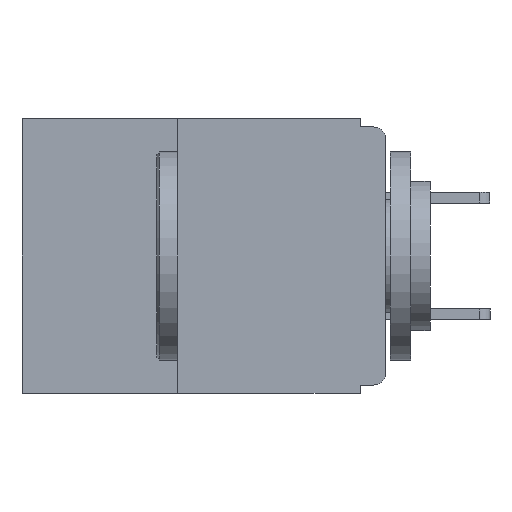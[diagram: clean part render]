
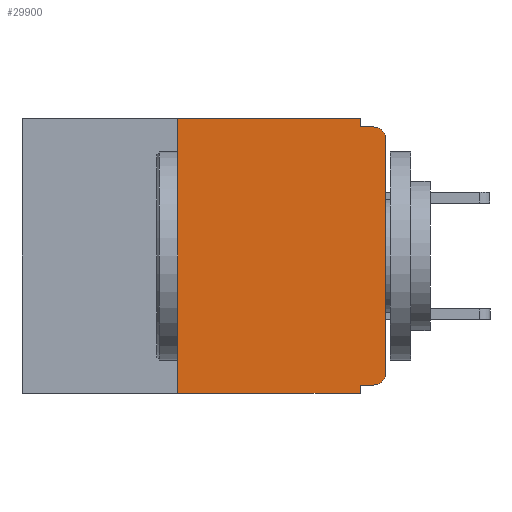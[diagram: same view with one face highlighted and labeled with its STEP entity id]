
A CAD part, left-side view. The second image highlights one B-rep face of the part: STEP entity #29900.
In plain terms, the highlighted planar face has unit normal (-1, 0, 0).
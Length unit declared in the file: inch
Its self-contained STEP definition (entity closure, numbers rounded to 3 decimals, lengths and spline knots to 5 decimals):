
#8 = CARTESIAN_POINT ( 'NONE',  ( 0., 0.031, -0.01 ) ) ;
#133 = CARTESIAN_POINT ( 'NONE',  ( 0., 0.031, 0. ) ) ;
#353 = CARTESIAN_POINT ( 'NONE',  ( 0., 0.437, 0. ) ) ;
#1776 = LINE ( 'NONE', #27268, #23215 ) ;
#1921 = EDGE_CURVE ( 'NONE', #31003, #8344, #16823, .T. ) ;
#2212 = LINE ( 'NONE', #31842, #16308 ) ;
#3171 = AXIS2_PLACEMENT_3D ( 'NONE', #21907, #5169, #24621 ) ;
#3263 = DIRECTION ( 'NONE',  ( 0., -1., 0. ) ) ;
#4074 = VERTEX_POINT ( 'NONE', #21590 ) ;
#4586 = CARTESIAN_POINT ( 'NONE',  ( 0., 0.25, 0. ) ) ;
#5169 = DIRECTION ( 'NONE',  ( -1., 0., 0. ) ) ;
#5334 = LINE ( 'NONE', #23595, #29151 ) ;
#5978 = CARTESIAN_POINT ( 'NONE',  ( 0., 0.437, 0. ) ) ;
#6447 = CARTESIAN_POINT ( 'NONE',  ( 0., 0.031, -0.32 ) ) ;
#6496 = VECTOR ( 'NONE', #3263, 39.37008 ) ;
#6951 = DIRECTION ( 'NONE',  ( 0., 0., -1. ) ) ;
#8344 = VERTEX_POINT ( 'NONE', #34713 ) ;
#8461 = VECTOR ( 'NONE', #34162, 39.37008 ) ;
#8498 = EDGE_CURVE ( 'NONE', #22569, #15946, #1776, .T. ) ;
#8713 = EDGE_CURVE ( 'NONE', #4074, #14890, #21919, .T. ) ;
#8714 = CARTESIAN_POINT ( 'NONE',  ( 0., 0.015, -0.32 ) ) ;
#8784 = DIRECTION ( 'NONE',  ( 0., 0., -1. ) ) ;
#9229 = AXIS2_PLACEMENT_3D ( 'NONE', #5978, #25416, #8784 ) ;
#9942 = VERTEX_POINT ( 'NONE', #30322 ) ;
#9954 = CARTESIAN_POINT ( 'NONE',  ( 0., 0.015, -0.305 ) ) ;
#10536 = ORIENTED_EDGE ( 'NONE', *, *, #19512, .T. ) ;
#11035 = ORIENTED_EDGE ( 'NONE', *, *, #20594, .F. ) ;
#12188 = EDGE_CURVE ( 'NONE', #9942, #26955, #2212, .T. ) ;
#12346 = EDGE_CURVE ( 'NONE', #4074, #24487, #34135, .T. ) ;
#12624 = DIRECTION ( 'NONE',  ( 0., 0., 1. ) ) ;
#12765 = DIRECTION ( 'NONE',  ( 0., 0., -1. ) ) ;
#13321 = CARTESIAN_POINT ( 'NONE',  ( 0., 0.437, -0.33 ) ) ;
#13657 = CARTESIAN_POINT ( 'NONE',  ( 0., 0.25, -0.33 ) ) ;
#13659 = ORIENTED_EDGE ( 'NONE', *, *, #26995, .F. ) ;
#14531 = VECTOR ( 'NONE', #12624, 39.37008 ) ;
#14890 = VERTEX_POINT ( 'NONE', #4586 ) ;
#15703 = ORIENTED_EDGE ( 'NONE', *, *, #1921, .F. ) ;
#15946 = VERTEX_POINT ( 'NONE', #6447 ) ;
#16308 = VECTOR ( 'NONE', #21122, 39.37008 ) ;
#16410 = CARTESIAN_POINT ( 'NONE',  ( 0., 0., -0.01 ) ) ;
#16823 = LINE ( 'NONE', #16410, #8461 ) ;
#17636 = ORIENTED_EDGE ( 'NONE', *, *, #12188, .T. ) ;
#19250 = VERTEX_POINT ( 'NONE', #133 ) ;
#19300 = ORIENTED_EDGE ( 'NONE', *, *, #8498, .F. ) ;
#19512 = EDGE_CURVE ( 'NONE', #22569, #9942, #28349, .T. ) ;
#19941 = PLANE ( 'NONE',  #9229 ) ;
#20594 = EDGE_CURVE ( 'NONE', #19250, #31003, #5334, .T. ) ;
#21122 = DIRECTION ( 'NONE',  ( 0., 0., 1. ) ) ;
#21481 = EDGE_CURVE ( 'NONE', #15946, #24487, #23580, .T. ) ;
#21590 = CARTESIAN_POINT ( 'NONE',  ( 0., 0.25, -0.33 ) ) ;
#21879 = VECTOR ( 'NONE', #28515, 39.37008 ) ;
#21907 = CARTESIAN_POINT ( 'NONE',  ( 0., 0.015, -0.025 ) ) ;
#21919 = LINE ( 'NONE', #13657, #14531 ) ;
#22569 = VERTEX_POINT ( 'NONE', #8714 ) ;
#22989 = ORIENTED_EDGE ( 'NONE', *, *, #12346, .T. ) ;
#23215 = VECTOR ( 'NONE', #28099, 39.37008 ) ;
#23580 = LINE ( 'NONE', #31158, #21879 ) ;
#23595 = CARTESIAN_POINT ( 'NONE',  ( 0., 0.031, 0. ) ) ;
#24487 = VERTEX_POINT ( 'NONE', #30721 ) ;
#24621 = DIRECTION ( 'NONE',  ( 0., 0., -1. ) ) ;
#25306 = CARTESIAN_POINT ( 'NONE',  ( 0., 0., -0.025 ) ) ;
#25416 = DIRECTION ( 'NONE',  ( 1., 0., 0. ) ) ;
#26684 = FACE_OUTER_BOUND ( 'NONE', #30454, .T. ) ;
#26955 = VERTEX_POINT ( 'NONE', #25306 ) ;
#26995 = EDGE_CURVE ( 'NONE', #14890, #19250, #28583, .T. ) ;
#27268 = CARTESIAN_POINT ( 'NONE',  ( 0., 0., -0.32 ) ) ;
#27946 = VECTOR ( 'NONE', #35082, 39.37008 ) ;
#28099 = DIRECTION ( 'NONE',  ( 0., 1., 0. ) ) ;
#28349 = CIRCLE ( 'NONE', #34639, 0.015 ) ;
#28515 = DIRECTION ( 'NONE',  ( 0., 0., -1. ) ) ;
#28583 = LINE ( 'NONE', #353, #6496 ) ;
#29151 = VECTOR ( 'NONE', #6951, 39.37008 ) ;
#29232 = DIRECTION ( 'NONE',  ( -1., 0., 0. ) ) ;
#29760 = CIRCLE ( 'NONE', #3171, 0.015 ) ;
#29900 = ADVANCED_FACE ( 'NONE', ( #26684 ), #19941, .F. ) ;
#30322 = CARTESIAN_POINT ( 'NONE',  ( 0., 0., -0.305 ) ) ;
#30454 = EDGE_LOOP ( 'NONE', ( #17636, #35126, #15703, #11035, #13659, #33135, #22989, #31436, #19300, #10536 ) ) ;
#30721 = CARTESIAN_POINT ( 'NONE',  ( 0., 0.031, -0.33 ) ) ;
#31003 = VERTEX_POINT ( 'NONE', #8 ) ;
#31158 = CARTESIAN_POINT ( 'NONE',  ( 0., 0.031, -0.33 ) ) ;
#31436 = ORIENTED_EDGE ( 'NONE', *, *, #21481, .F. ) ;
#31842 = CARTESIAN_POINT ( 'NONE',  ( 0., 0., 0. ) ) ;
#33135 = ORIENTED_EDGE ( 'NONE', *, *, #8713, .F. ) ;
#33825 = EDGE_CURVE ( 'NONE', #26955, #8344, #29760, .T. ) ;
#34135 = LINE ( 'NONE', #13321, #27946 ) ;
#34162 = DIRECTION ( 'NONE',  ( 0., -1., 0. ) ) ;
#34639 = AXIS2_PLACEMENT_3D ( 'NONE', #9954, #29232, #12765 ) ;
#34713 = CARTESIAN_POINT ( 'NONE',  ( 0., 0.015, -0.01 ) ) ;
#35082 = DIRECTION ( 'NONE',  ( 0., -1., 0. ) ) ;
#35126 = ORIENTED_EDGE ( 'NONE', *, *, #33825, .T. ) ;
